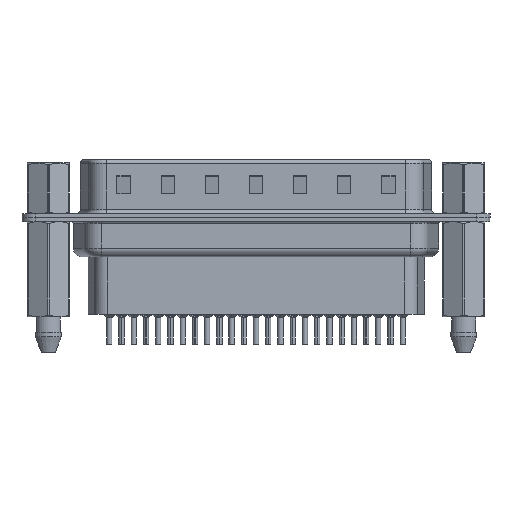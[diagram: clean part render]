
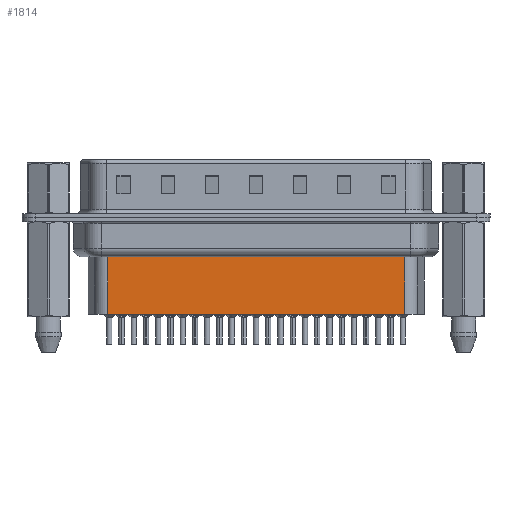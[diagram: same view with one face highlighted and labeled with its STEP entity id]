
A CAD part, front view. The second image highlights one B-rep face of the part: STEP entity #1814.
In plain terms, the highlighted planar face has unit normal (0, -1, 0).
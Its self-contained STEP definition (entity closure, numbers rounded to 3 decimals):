
#1302 = EDGE_CURVE ( 'NONE', #11022, #14927, #24855, .T. ) ;
#1655 = CARTESIAN_POINT ( 'NONE',  ( 6.459, -3.5, -4.097 ) ) ;
#1814 = ADVANCED_FACE ( 'NONE', ( #26436 ), #5587, .T. ) ;
#3814 = EDGE_CURVE ( 'NONE', #30764, #22927, #16359, .T. ) ;
#5587 = PLANE ( 'NONE',  #29731 ) ;
#6250 = CARTESIAN_POINT ( 'NONE',  ( 40.344, -3.5, -4.097 ) ) ;
#6690 = ORIENTED_EDGE ( 'NONE', *, *, #13392, .T. ) ;
#6947 = CARTESIAN_POINT ( 'NONE',  ( 40.344, -3.5, -10.95 ) ) ;
#8621 = CARTESIAN_POINT ( 'NONE',  ( 40.344, -3.5, -3.1 ) ) ;
#10676 = VECTOR ( 'NONE', #29180, 1000. ) ;
#11022 = VERTEX_POINT ( 'NONE', #6250 ) ;
#12515 = EDGE_CURVE ( 'NONE', #11022, #30764, #13826, .T. ) ;
#12866 = VECTOR ( 'NONE', #26469, 1000. ) ;
#13392 = EDGE_CURVE ( 'NONE', #14927, #22927, #32186, .T. ) ;
#13826 = LINE ( 'NONE', #8621, #10676 ) ;
#14927 = VERTEX_POINT ( 'NONE', #28905 ) ;
#15705 = CARTESIAN_POINT ( 'NONE',  ( 6.706, -3.5, -10.95 ) ) ;
#15834 = DIRECTION ( 'NONE',  ( 0., -1., 0. ) ) ;
#16096 = ORIENTED_EDGE ( 'NONE', *, *, #12515, .F. ) ;
#16310 = ORIENTED_EDGE ( 'NONE', *, *, #3814, .F. ) ;
#16359 = LINE ( 'NONE', #31380, #22139 ) ;
#18511 = CARTESIAN_POINT ( 'NONE',  ( 6.706, -3.5, -3.1 ) ) ;
#18559 = EDGE_LOOP ( 'NONE', ( #16096, #26979, #6690, #16310 ) ) ;
#19198 = DIRECTION ( 'NONE',  ( -1., 0., 0. ) ) ;
#21158 = VECTOR ( 'NONE', #22301, 1000. ) ;
#22139 = VECTOR ( 'NONE', #19198, 1000. ) ;
#22301 = DIRECTION ( 'NONE',  ( -1., 0., 0. ) ) ;
#22927 = VERTEX_POINT ( 'NONE', #15705 ) ;
#24855 = LINE ( 'NONE', #1655, #21158 ) ;
#26436 = FACE_OUTER_BOUND ( 'NONE', #18559, .T. ) ;
#26469 = DIRECTION ( 'NONE',  ( 0., 0., -1. ) ) ;
#26979 = ORIENTED_EDGE ( 'NONE', *, *, #1302, .T. ) ;
#28905 = CARTESIAN_POINT ( 'NONE',  ( 6.706, -3.5, -4.097 ) ) ;
#29180 = DIRECTION ( 'NONE',  ( 0., 0., -1. ) ) ;
#29344 = CARTESIAN_POINT ( 'NONE',  ( 6.706, -3.5, -3.1 ) ) ;
#29731 = AXIS2_PLACEMENT_3D ( 'NONE', #18511, #15834, #31493 ) ;
#30764 = VERTEX_POINT ( 'NONE', #6947 ) ;
#31380 = CARTESIAN_POINT ( 'NONE',  ( 6.706, -3.5, -10.95 ) ) ;
#31493 = DIRECTION ( 'NONE',  ( 1., 0., 0. ) ) ;
#32186 = LINE ( 'NONE', #29344, #12866 ) ;
